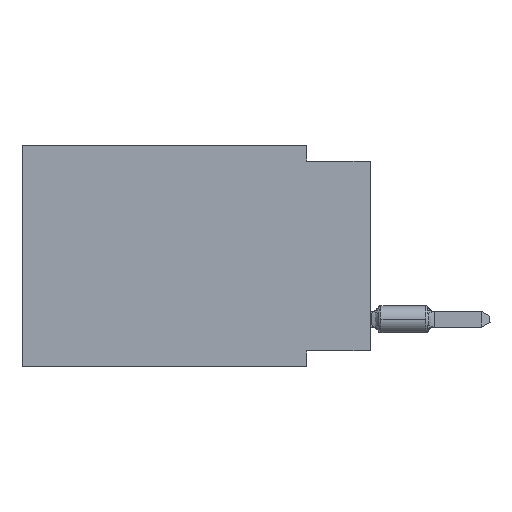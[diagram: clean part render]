
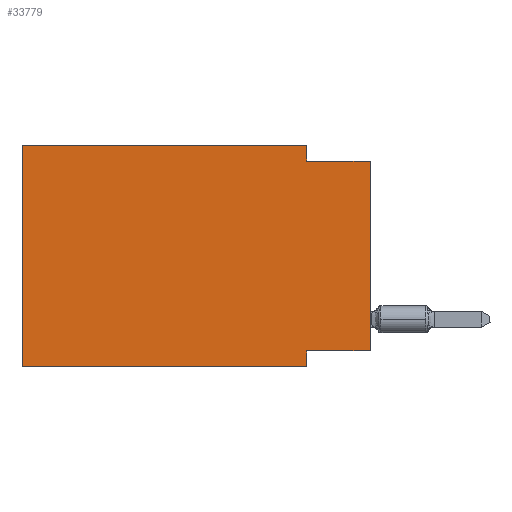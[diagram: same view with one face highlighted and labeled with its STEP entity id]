
A CAD part, left-side view. The second image highlights one B-rep face of the part: STEP entity #33779.
In plain terms, the highlighted planar face has unit normal (-1, 0, 0).
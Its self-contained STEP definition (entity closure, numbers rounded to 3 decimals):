
#240 = VECTOR ( 'NONE', #45162, 1000. ) ;
#428 = LINE ( 'NONE', #40473, #240 ) ;
#1408 = EDGE_CURVE ( 'NONE', #48893, #17007, #30007, .T. ) ;
#2123 = VERTEX_POINT ( 'NONE', #9741 ) ;
#3657 = CARTESIAN_POINT ( 'NONE',  ( 0., 2.54, -8.89 ) ) ;
#6897 = ORIENTED_EDGE ( 'NONE', *, *, #17999, .F. ) ;
#7425 = CARTESIAN_POINT ( 'NONE',  ( 0., 2.54, -0.635 ) ) ;
#7938 = DIRECTION ( 'NONE',  ( 0., 1., 0. ) ) ;
#8058 = EDGE_CURVE ( 'NONE', #42943, #47426, #60675, .T. ) ;
#8728 = LINE ( 'NONE', #64191, #59652 ) ;
#9741 = CARTESIAN_POINT ( 'NONE',  ( 0., 13.97, -8.89 ) ) ;
#9749 = CARTESIAN_POINT ( 'NONE',  ( 0., 0., 0. ) ) ;
#9799 = ORIENTED_EDGE ( 'NONE', *, *, #65654, .F. ) ;
#9910 = VECTOR ( 'NONE', #65983, 1000. ) ;
#12599 = DIRECTION ( 'NONE',  ( 1., 0., 0. ) ) ;
#12912 = CARTESIAN_POINT ( 'NONE',  ( 0., 0., -8.255 ) ) ;
#13650 = EDGE_CURVE ( 'NONE', #30395, #15715, #21066, .T. ) ;
#13707 = CARTESIAN_POINT ( 'NONE',  ( 0., 2.54, 0. ) ) ;
#15263 = EDGE_CURVE ( 'NONE', #46042, #15715, #8728, .T. ) ;
#15296 = ORIENTED_EDGE ( 'NONE', *, *, #8058, .F. ) ;
#15715 = VERTEX_POINT ( 'NONE', #59984 ) ;
#15822 = VECTOR ( 'NONE', #56684, 1000. ) ;
#17007 = VERTEX_POINT ( 'NONE', #52810 ) ;
#17614 = ORIENTED_EDGE ( 'NONE', *, *, #35115, .F. ) ;
#17999 = EDGE_CURVE ( 'NONE', #2123, #42943, #60302, .T. ) ;
#21066 = LINE ( 'NONE', #9749, #44301 ) ;
#22296 = PLANE ( 'NONE',  #36251 ) ;
#23739 = VECTOR ( 'NONE', #34073, 1000. ) ;
#23861 = VECTOR ( 'NONE', #7938, 1000. ) ;
#24810 = ORIENTED_EDGE ( 'NONE', *, *, #15263, .F. ) ;
#25623 = CARTESIAN_POINT ( 'NONE',  ( 0., 13.97, 0. ) ) ;
#26094 = DIRECTION ( 'NONE',  ( 0., 0., 1. ) ) ;
#28615 = CARTESIAN_POINT ( 'NONE',  ( 0., 13.97, 0. ) ) ;
#30007 = LINE ( 'NONE', #3657, #39205 ) ;
#30395 = VERTEX_POINT ( 'NONE', #12912 ) ;
#30638 = DIRECTION ( 'NONE',  ( 0., -1., 0. ) ) ;
#33325 = DIRECTION ( 'NONE',  ( 0., 0., -1. ) ) ;
#33335 = CARTESIAN_POINT ( 'NONE',  ( 0., 0., -8.255 ) ) ;
#33779 = ADVANCED_FACE ( 'NONE', ( #47658 ), #22296, .F. ) ;
#34073 = DIRECTION ( 'NONE',  ( 0., 0., -1. ) ) ;
#34262 = EDGE_LOOP ( 'NONE', ( #48182, #24810, #9799, #15296, #6897, #41048, #53675, #17614 ) ) ;
#35115 = EDGE_CURVE ( 'NONE', #30395, #48893, #64390, .T. ) ;
#36251 = AXIS2_PLACEMENT_3D ( 'NONE', #28615, #12599, #33325 ) ;
#39205 = VECTOR ( 'NONE', #54053, 1000. ) ;
#39754 = LINE ( 'NONE', #13707, #23739 ) ;
#39876 = CARTESIAN_POINT ( 'NONE',  ( 0., 2.54, 0. ) ) ;
#40473 = CARTESIAN_POINT ( 'NONE',  ( 0., 13.97, -8.89 ) ) ;
#41048 = ORIENTED_EDGE ( 'NONE', *, *, #63715, .T. ) ;
#42943 = VERTEX_POINT ( 'NONE', #60110 ) ;
#44301 = VECTOR ( 'NONE', #26094, 1000. ) ;
#45162 = DIRECTION ( 'NONE',  ( 0., -1., 0. ) ) ;
#46042 = VERTEX_POINT ( 'NONE', #7425 ) ;
#47426 = VERTEX_POINT ( 'NONE', #39876 ) ;
#47658 = FACE_OUTER_BOUND ( 'NONE', #34262, .T. ) ;
#48182 = ORIENTED_EDGE ( 'NONE', *, *, #13650, .T. ) ;
#48893 = VERTEX_POINT ( 'NONE', #65376 ) ;
#50601 = CARTESIAN_POINT ( 'NONE',  ( 0., 13.97, 0. ) ) ;
#52810 = CARTESIAN_POINT ( 'NONE',  ( 0., 2.54, -8.89 ) ) ;
#53675 = ORIENTED_EDGE ( 'NONE', *, *, #1408, .F. ) ;
#54053 = DIRECTION ( 'NONE',  ( 0., 0., -1. ) ) ;
#56684 = DIRECTION ( 'NONE',  ( 0., -1., 0. ) ) ;
#59652 = VECTOR ( 'NONE', #30638, 1000. ) ;
#59984 = CARTESIAN_POINT ( 'NONE',  ( 0., 0., -0.635 ) ) ;
#60110 = CARTESIAN_POINT ( 'NONE',  ( 0., 13.97, 0. ) ) ;
#60302 = LINE ( 'NONE', #50601, #9910 ) ;
#60675 = LINE ( 'NONE', #25623, #15822 ) ;
#63715 = EDGE_CURVE ( 'NONE', #2123, #17007, #428, .T. ) ;
#64191 = CARTESIAN_POINT ( 'NONE',  ( 0., 0., -0.635 ) ) ;
#64390 = LINE ( 'NONE', #33335, #23861 ) ;
#65376 = CARTESIAN_POINT ( 'NONE',  ( 0., 2.54, -8.255 ) ) ;
#65654 = EDGE_CURVE ( 'NONE', #47426, #46042, #39754, .T. ) ;
#65983 = DIRECTION ( 'NONE',  ( 0., 0., 1. ) ) ;
